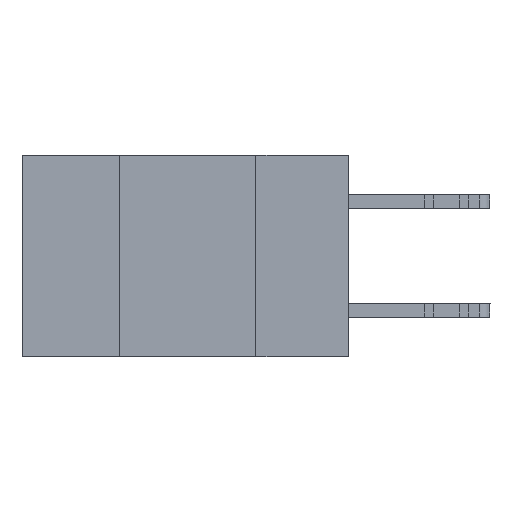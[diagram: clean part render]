
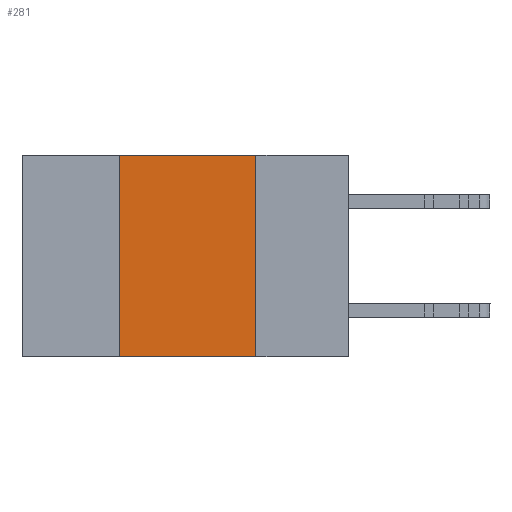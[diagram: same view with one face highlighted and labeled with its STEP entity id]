
A CAD part, left-side view. The second image highlights one B-rep face of the part: STEP entity #281.
In plain terms, the highlighted planar face has unit normal (-1, 0, 0).
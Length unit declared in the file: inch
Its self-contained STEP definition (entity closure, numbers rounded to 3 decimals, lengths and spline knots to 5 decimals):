
#281 = ADVANCED_FACE ( 'NONE', ( #24649 ), #6014, .F. ) ;
#904 = EDGE_CURVE ( 'NONE', #14154, #19264, #11818, .T. ) ;
#996 = EDGE_LOOP ( 'NONE', ( #5245, #12430, #1961, #12107 ) ) ;
#1961 = ORIENTED_EDGE ( 'NONE', *, *, #904, .F. ) ;
#2842 = EDGE_CURVE ( 'NONE', #14154, #26703, #16820, .T. ) ;
#4598 = CARTESIAN_POINT ( 'NONE',  ( 0., 0.6, 0. ) ) ;
#4743 = VECTOR ( 'NONE', #25142, 39.37008 ) ;
#5245 = ORIENTED_EDGE ( 'NONE', *, *, #13489, .F. ) ;
#5863 = DIRECTION ( 'NONE',  ( 0., 0., -1. ) ) ;
#5943 = DIRECTION ( 'NONE',  ( 1., 0., 0. ) ) ;
#6014 = PLANE ( 'NONE',  #23125 ) ;
#6402 = CARTESIAN_POINT ( 'NONE',  ( 0., 0.6, 0. ) ) ;
#7933 = EDGE_CURVE ( 'NONE', #19264, #24696, #21138, .T. ) ;
#9510 = VECTOR ( 'NONE', #21174, 39.37008 ) ;
#9692 = CARTESIAN_POINT ( 'NONE',  ( 0., 0.42, 0. ) ) ;
#10270 = CARTESIAN_POINT ( 'NONE',  ( 0., 0.42, -0.37 ) ) ;
#11226 = DIRECTION ( 'NONE',  ( 0., 0., 1. ) ) ;
#11818 = LINE ( 'NONE', #10270, #15334 ) ;
#12107 = ORIENTED_EDGE ( 'NONE', *, *, #2842, .T. ) ;
#12430 = ORIENTED_EDGE ( 'NONE', *, *, #7933, .F. ) ;
#13489 = EDGE_CURVE ( 'NONE', #24696, #26703, #26645, .T. ) ;
#14154 = VERTEX_POINT ( 'NONE', #16969 ) ;
#15334 = VECTOR ( 'NONE', #11226, 39.37008 ) ;
#16820 = LINE ( 'NONE', #20069, #21683 ) ;
#16969 = CARTESIAN_POINT ( 'NONE',  ( 0., 0.42, -0.37 ) ) ;
#18540 = CARTESIAN_POINT ( 'NONE',  ( 0., 0.17, 0. ) ) ;
#19264 = VERTEX_POINT ( 'NONE', #9692 ) ;
#19946 = DIRECTION ( 'NONE',  ( 0., -1., 0. ) ) ;
#20069 = CARTESIAN_POINT ( 'NONE',  ( 0., 0.6, -0.37 ) ) ;
#21138 = LINE ( 'NONE', #4598, #9510 ) ;
#21174 = DIRECTION ( 'NONE',  ( 0., -1., 0. ) ) ;
#21683 = VECTOR ( 'NONE', #19946, 39.37008 ) ;
#23108 = CARTESIAN_POINT ( 'NONE',  ( 0., 0.17, -0.37 ) ) ;
#23125 = AXIS2_PLACEMENT_3D ( 'NONE', #6402, #5943, #5863 ) ;
#24135 = CARTESIAN_POINT ( 'NONE',  ( 0., 0.17, -0.37 ) ) ;
#24649 = FACE_OUTER_BOUND ( 'NONE', #996, .T. ) ;
#24696 = VERTEX_POINT ( 'NONE', #18540 ) ;
#25142 = DIRECTION ( 'NONE',  ( 0., 0., -1. ) ) ;
#26645 = LINE ( 'NONE', #23108, #4743 ) ;
#26703 = VERTEX_POINT ( 'NONE', #24135 ) ;
